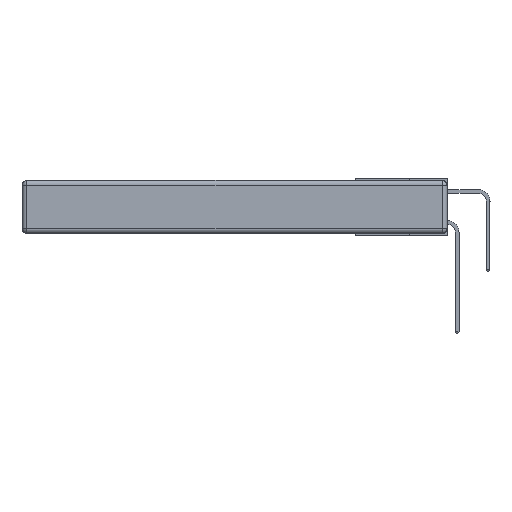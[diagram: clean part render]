
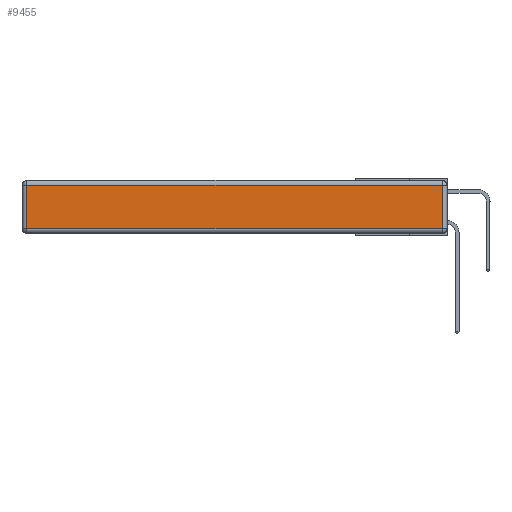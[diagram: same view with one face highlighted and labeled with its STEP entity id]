
A CAD part, left-side view. The second image highlights one B-rep face of the part: STEP entity #9455.
In plain terms, the highlighted planar face has unit normal (-1, 0, 0).
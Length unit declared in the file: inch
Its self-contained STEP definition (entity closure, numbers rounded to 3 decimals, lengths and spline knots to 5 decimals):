
#811 = EDGE_CURVE ( 'NONE', #9376, #11773, #4163, .T. ) ;
#1713 = DIRECTION ( 'NONE',  ( 0., 0., 1. ) ) ;
#1842 = DIRECTION ( 'NONE',  ( 0., -1., 0. ) ) ;
#3820 = LINE ( 'NONE', #8550, #4512 ) ;
#4163 = LINE ( 'NONE', #17394, #23314 ) ;
#4512 = VECTOR ( 'NONE', #1842, 39.37008 ) ;
#5404 = DIRECTION ( 'NONE',  ( 0., 0., -1. ) ) ;
#6606 = CARTESIAN_POINT ( 'NONE',  ( 0., 2.72, -0.03 ) ) ;
#6906 = CARTESIAN_POINT ( 'NONE',  ( 0., 0.03, -0.03 ) ) ;
#8193 = CARTESIAN_POINT ( 'NONE',  ( 0., 0.03, -0.313 ) ) ;
#8550 = CARTESIAN_POINT ( 'NONE',  ( 0., 0., -0.313 ) ) ;
#9376 = VERTEX_POINT ( 'NONE', #8193 ) ;
#9455 = ADVANCED_FACE ( 'NONE', ( #16651 ), #13101, .T. ) ;
#9587 = VERTEX_POINT ( 'NONE', #6606 ) ;
#10252 = AXIS2_PLACEMENT_3D ( 'NONE', #24131, #17356, #26530 ) ;
#11773 = VERTEX_POINT ( 'NONE', #6906 ) ;
#13101 = PLANE ( 'NONE',  #10252 ) ;
#13809 = EDGE_CURVE ( 'NONE', #9587, #21156, #24571, .T. ) ;
#15709 = CARTESIAN_POINT ( 'NONE',  ( 0., 2.75, -0.03 ) ) ;
#15813 = DIRECTION ( 'NONE',  ( 0., 1., 0. ) ) ;
#16602 = CARTESIAN_POINT ( 'NONE',  ( 0., 2.72, -0.343 ) ) ;
#16651 = FACE_OUTER_BOUND ( 'NONE', #23368, .T. ) ;
#17112 = ORIENTED_EDGE ( 'NONE', *, *, #811, .T. ) ;
#17356 = DIRECTION ( 'NONE',  ( -1., 0., 0. ) ) ;
#17394 = CARTESIAN_POINT ( 'NONE',  ( 0., 0.03, -0.343 ) ) ;
#18009 = VECTOR ( 'NONE', #5404, 39.37008 ) ;
#18157 = VECTOR ( 'NONE', #15813, 39.37008 ) ;
#18796 = EDGE_CURVE ( 'NONE', #21156, #9376, #3820, .T. ) ;
#21156 = VERTEX_POINT ( 'NONE', #26920 ) ;
#21376 = ORIENTED_EDGE ( 'NONE', *, *, #23195, .T. ) ;
#23195 = EDGE_CURVE ( 'NONE', #11773, #9587, #25750, .T. ) ;
#23314 = VECTOR ( 'NONE', #1713, 39.37008 ) ;
#23368 = EDGE_LOOP ( 'NONE', ( #25652, #17112, #21376, #25800 ) ) ;
#24131 = CARTESIAN_POINT ( 'NONE',  ( 0., 0., -0.343 ) ) ;
#24571 = LINE ( 'NONE', #16602, #18009 ) ;
#25652 = ORIENTED_EDGE ( 'NONE', *, *, #18796, .T. ) ;
#25750 = LINE ( 'NONE', #15709, #18157 ) ;
#25800 = ORIENTED_EDGE ( 'NONE', *, *, #13809, .T. ) ;
#26530 = DIRECTION ( 'NONE',  ( 0., 0., 1. ) ) ;
#26920 = CARTESIAN_POINT ( 'NONE',  ( 0., 2.72, -0.313 ) ) ;
